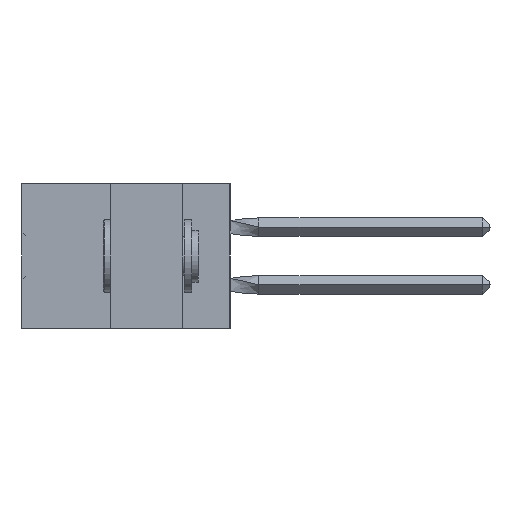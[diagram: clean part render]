
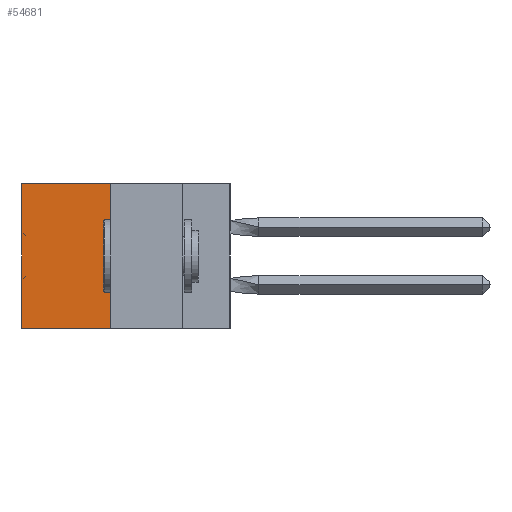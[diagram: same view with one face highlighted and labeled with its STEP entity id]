
A CAD part, left-side view. The second image highlights one B-rep face of the part: STEP entity #54681.
In plain terms, the highlighted planar face has unit normal (-1, 0, 0).
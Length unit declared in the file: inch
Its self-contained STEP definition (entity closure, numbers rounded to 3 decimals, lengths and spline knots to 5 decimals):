
#509 = CARTESIAN_POINT ( 'NONE',  ( 0.305, 0.72, -0.5 ) ) ;
#1369 = VERTEX_POINT ( 'NONE', #54978 ) ;
#5581 = VERTEX_POINT ( 'NONE', #39133 ) ;
#9588 = DIRECTION ( 'NONE',  ( 0., 0., -1. ) ) ;
#13366 = VERTEX_POINT ( 'NONE', #42248 ) ;
#14221 = DIRECTION ( 'NONE',  ( 0., 1., 0. ) ) ;
#15552 = CARTESIAN_POINT ( 'NONE',  ( 0.305, 0.413, -0.5 ) ) ;
#16047 = VECTOR ( 'NONE', #54501, 39.37008 ) ;
#16388 = EDGE_CURVE ( 'NONE', #1369, #5581, #35024, .T. ) ;
#16779 = LINE ( 'NONE', #37083, #16047 ) ;
#17260 = CARTESIAN_POINT ( 'NONE',  ( 0.305, 0.413, -0.5 ) ) ;
#17590 = VECTOR ( 'NONE', #35260, 39.37008 ) ;
#18419 = CARTESIAN_POINT ( 'NONE',  ( 0.305, 0.413, 0. ) ) ;
#21478 = VECTOR ( 'NONE', #9588, 39.37008 ) ;
#22875 = ORIENTED_EDGE ( 'NONE', *, *, #57328, .F. ) ;
#27253 = EDGE_CURVE ( 'NONE', #13366, #1369, #52488, .T. ) ;
#28095 = PLANE ( 'NONE',  #30056 ) ;
#29067 = DIRECTION ( 'NONE',  ( 1., 0., 0. ) ) ;
#30056 = AXIS2_PLACEMENT_3D ( 'NONE', #15552, #29067, #56447 ) ;
#35024 = LINE ( 'NONE', #509, #21478 ) ;
#35260 = DIRECTION ( 'NONE',  ( 0., 1., 0. ) ) ;
#36113 = ORIENTED_EDGE ( 'NONE', *, *, #27253, .T. ) ;
#36327 = EDGE_LOOP ( 'NONE', ( #58268, #22875, #40100, #36113 ) ) ;
#37083 = CARTESIAN_POINT ( 'NONE',  ( 0.305, 0.413, -0.5 ) ) ;
#39133 = CARTESIAN_POINT ( 'NONE',  ( 0.305, 0.72, -0.5 ) ) ;
#39850 = EDGE_CURVE ( 'NONE', #13366, #44143, #16779, .T. ) ;
#40100 = ORIENTED_EDGE ( 'NONE', *, *, #39850, .F. ) ;
#42248 = CARTESIAN_POINT ( 'NONE',  ( 0.305, 0.413, 0. ) ) ;
#44143 = VERTEX_POINT ( 'NONE', #17260 ) ;
#50972 = LINE ( 'NONE', #51935, #17590 ) ;
#51935 = CARTESIAN_POINT ( 'NONE',  ( 0.305, 0.413, -0.5 ) ) ;
#52488 = LINE ( 'NONE', #18419, #56050 ) ;
#54501 = DIRECTION ( 'NONE',  ( 0., 0., -1. ) ) ;
#54681 = ADVANCED_FACE ( 'NONE', ( #55522 ), #28095, .F. ) ;
#54978 = CARTESIAN_POINT ( 'NONE',  ( 0.305, 0.72, 0. ) ) ;
#55522 = FACE_OUTER_BOUND ( 'NONE', #36327, .T. ) ;
#56050 = VECTOR ( 'NONE', #14221, 39.37008 ) ;
#56447 = DIRECTION ( 'NONE',  ( 0., 0., -1. ) ) ;
#57328 = EDGE_CURVE ( 'NONE', #44143, #5581, #50972, .T. ) ;
#58268 = ORIENTED_EDGE ( 'NONE', *, *, #16388, .T. ) ;
